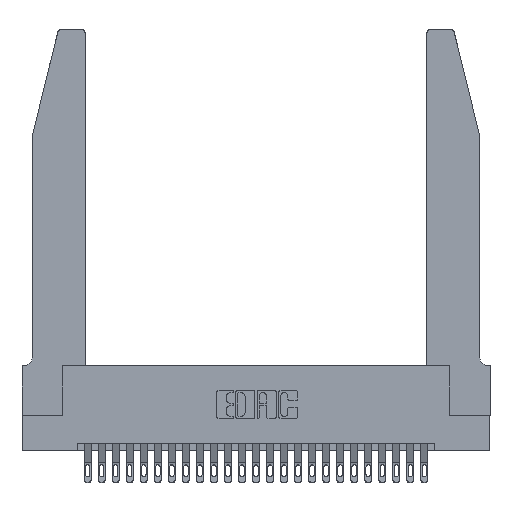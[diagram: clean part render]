
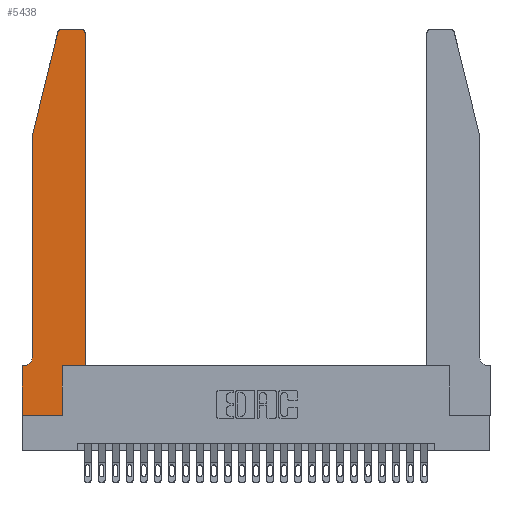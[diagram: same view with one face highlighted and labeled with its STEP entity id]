
A CAD part, top view. The second image highlights one B-rep face of the part: STEP entity #5438.
In plain terms, the highlighted planar face has unit normal (0, 0, 1).
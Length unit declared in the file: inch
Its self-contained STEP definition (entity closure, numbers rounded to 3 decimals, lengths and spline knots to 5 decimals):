
#113 = EDGE_CURVE ( 'NONE', #25436, #23786, #5286, .T. ) ;
#147 = EDGE_CURVE ( 'NONE', #23786, #20704, #4611, .T. ) ;
#660 = CARTESIAN_POINT ( 'NONE',  ( 0.284, 2.75, 0.37 ) ) ;
#758 = VECTOR ( 'NONE', #20936, 39.37008 ) ;
#1079 = PLANE ( 'NONE',  #24748 ) ;
#1210 = VERTEX_POINT ( 'NONE', #26761 ) ;
#1295 = AXIS2_PLACEMENT_3D ( 'NONE', #12065, #11718, #9719 ) ;
#1422 = FACE_OUTER_BOUND ( 'NONE', #10379, .T. ) ;
#1890 = VERTEX_POINT ( 'NONE', #9913 ) ;
#2035 = ORIENTED_EDGE ( 'NONE', *, *, #22057, .T. ) ;
#2702 = LINE ( 'NONE', #21032, #758 ) ;
#2763 = DIRECTION ( 'NONE',  ( 0., 1., 0. ) ) ;
#2892 = CARTESIAN_POINT ( 'NONE',  ( 0., 0., 0.37 ) ) ;
#3364 = ORIENTED_EDGE ( 'NONE', *, *, #16850, .T. ) ;
#3591 = DIRECTION ( 'NONE',  ( -1., 0., 0. ) ) ;
#3679 = CARTESIAN_POINT ( 'NONE',  ( 0., 0., 0.37 ) ) ;
#3851 = DIRECTION ( 'NONE',  ( 1., 0., 0. ) ) ;
#3941 = DIRECTION ( 'NONE',  ( 0., 0., 1. ) ) ;
#4061 = LINE ( 'NONE', #22363, #6693 ) ;
#4368 = LINE ( 'NONE', #18089, #11891 ) ;
#4611 = LINE ( 'NONE', #3679, #24851 ) ;
#5286 = LINE ( 'NONE', #16263, #26804 ) ;
#5438 = ADVANCED_FACE ( 'NONE', ( #1422 ), #1079, .T. ) ;
#6693 = VECTOR ( 'NONE', #19968, 39.37008 ) ;
#6712 = VECTOR ( 'NONE', #13705, 39.37008 ) ;
#7265 = ORIENTED_EDGE ( 'NONE', *, *, #12050, .T. ) ;
#7304 = CARTESIAN_POINT ( 'NONE',  ( 0.2865, 0., 0.37 ) ) ;
#7962 = CARTESIAN_POINT ( 'NONE',  ( 0.2865, 0.35, 0.37 ) ) ;
#8316 = CARTESIAN_POINT ( 'NONE',  ( 0.0755, 2., 0.37 ) ) ;
#8392 = VERTEX_POINT ( 'NONE', #660 ) ;
#9274 = CIRCLE ( 'NONE', #1295, 0.07 ) ;
#9284 = CARTESIAN_POINT ( 'NONE',  ( 0., 0.35, 0.37 ) ) ;
#9291 = DIRECTION ( 'NONE',  ( 1., 0., 0. ) ) ;
#9356 = EDGE_CURVE ( 'NONE', #17501, #8392, #16219, .T. ) ;
#9461 = DIRECTION ( 'NONE',  ( 1., 0., 0. ) ) ;
#9602 = VERTEX_POINT ( 'NONE', #13536 ) ;
#9719 = DIRECTION ( 'NONE',  ( -1., 0., 0. ) ) ;
#9913 = CARTESIAN_POINT ( 'NONE',  ( 0.0755, 2., 0.37 ) ) ;
#9938 = LINE ( 'NONE', #15140, #16427 ) ;
#10162 = CARTESIAN_POINT ( 'NONE',  ( 0.4205, 2.72, 0.37 ) ) ;
#10234 = CIRCLE ( 'NONE', #24543, 0.03 ) ;
#10379 = EDGE_LOOP ( 'NONE', ( #18372, #12619, #7265, #15109, #2035, #25795, #15486, #26771, #3364, #12554, #19840, #25245 ) ) ;
#10765 = VERTEX_POINT ( 'NONE', #7962 ) ;
#11630 = CARTESIAN_POINT ( 'NONE',  ( 0.0755, 2., 0.37 ) ) ;
#11718 = DIRECTION ( 'NONE',  ( 0., 0., -1. ) ) ;
#11820 = CARTESIAN_POINT ( 'NONE',  ( 0.0055, 0.35, 0.37 ) ) ;
#11891 = VECTOR ( 'NONE', #22448, 39.37008 ) ;
#12050 = EDGE_CURVE ( 'NONE', #9602, #1890, #23351, .T. ) ;
#12065 = CARTESIAN_POINT ( 'NONE',  ( 0.0055, 0.42, 0.37 ) ) ;
#12495 = EDGE_CURVE ( 'NONE', #1210, #14931, #9938, .T. ) ;
#12554 = ORIENTED_EDGE ( 'NONE', *, *, #21561, .T. ) ;
#12619 = ORIENTED_EDGE ( 'NONE', *, *, #13758, .T. ) ;
#12656 = VECTOR ( 'NONE', #12910, 39.37008 ) ;
#12910 = DIRECTION ( 'NONE',  ( -1., 0., 0. ) ) ;
#13092 = CARTESIAN_POINT ( 'NONE',  ( 0.2605, 2.75, 0.37 ) ) ;
#13536 = CARTESIAN_POINT ( 'NONE',  ( 0.25487, 2.72718, 0.37 ) ) ;
#13632 = DIRECTION ( 'NONE',  ( 0., 0., 1. ) ) ;
#13705 = DIRECTION ( 'NONE',  ( -0.239, -0.971, 0. ) ) ;
#13758 = EDGE_CURVE ( 'NONE', #8392, #9602, #10234, .T. ) ;
#14931 = VERTEX_POINT ( 'NONE', #19431 ) ;
#15109 = ORIENTED_EDGE ( 'NONE', *, *, #22905, .T. ) ;
#15140 = CARTESIAN_POINT ( 'NONE',  ( 0.4505, 0.35, 0.37 ) ) ;
#15486 = ORIENTED_EDGE ( 'NONE', *, *, #147, .T. ) ;
#15714 = DIRECTION ( 'NONE',  ( 0., 0., 1. ) ) ;
#16219 = LINE ( 'NONE', #13092, #12656 ) ;
#16263 = CARTESIAN_POINT ( 'NONE',  ( 0.0755, 0.35, 0.37 ) ) ;
#16415 = VERTEX_POINT ( 'NONE', #7304 ) ;
#16427 = VECTOR ( 'NONE', #2763, 39.37008 ) ;
#16850 = EDGE_CURVE ( 'NONE', #16415, #10765, #2702, .T. ) ;
#17501 = VERTEX_POINT ( 'NONE', #18637 ) ;
#17822 = VECTOR ( 'NONE', #22817, 39.37008 ) ;
#18089 = CARTESIAN_POINT ( 'NONE',  ( 0.4505, 0.35, 0.37 ) ) ;
#18372 = ORIENTED_EDGE ( 'NONE', *, *, #9356, .T. ) ;
#18637 = CARTESIAN_POINT ( 'NONE',  ( 0.4205, 2.75, 0.37 ) ) ;
#18761 = VERTEX_POINT ( 'NONE', #25028 ) ;
#19119 = AXIS2_PLACEMENT_3D ( 'NONE', #10162, #3941, #3851 ) ;
#19431 = CARTESIAN_POINT ( 'NONE',  ( 0.4505, 2.72, 0.37 ) ) ;
#19840 = ORIENTED_EDGE ( 'NONE', *, *, #12495, .T. ) ;
#19968 = DIRECTION ( 'NONE',  ( 1., 0., 0. ) ) ;
#20704 = VERTEX_POINT ( 'NONE', #2892 ) ;
#20936 = DIRECTION ( 'NONE',  ( 0., 1., 0. ) ) ;
#21032 = CARTESIAN_POINT ( 'NONE',  ( 0.2865, 0.35, 0.37 ) ) ;
#21454 = EDGE_CURVE ( 'NONE', #20704, #16415, #4061, .T. ) ;
#21561 = EDGE_CURVE ( 'NONE', #10765, #1210, #4368, .T. ) ;
#21776 = CARTESIAN_POINT ( 'NONE',  ( 0.284, 2.72, 0.37 ) ) ;
#22057 = EDGE_CURVE ( 'NONE', #18761, #25436, #9274, .T. ) ;
#22363 = CARTESIAN_POINT ( 'NONE',  ( 0., 0., 0.37 ) ) ;
#22448 = DIRECTION ( 'NONE',  ( 1., 0., 0. ) ) ;
#22681 = DIRECTION ( 'NONE',  ( 0., -1., 0. ) ) ;
#22817 = DIRECTION ( 'NONE',  ( 0., -1., 0. ) ) ;
#22905 = EDGE_CURVE ( 'NONE', #1890, #18761, #26264, .T. ) ;
#23351 = LINE ( 'NONE', #11630, #6712 ) ;
#23678 = CARTESIAN_POINT ( 'NONE',  ( 0., 0.35, 0.37 ) ) ;
#23786 = VERTEX_POINT ( 'NONE', #23678 ) ;
#24008 = EDGE_CURVE ( 'NONE', #14931, #17501, #25578, .T. ) ;
#24543 = AXIS2_PLACEMENT_3D ( 'NONE', #21776, #13632, #9291 ) ;
#24748 = AXIS2_PLACEMENT_3D ( 'NONE', #9284, #15714, #9461 ) ;
#24851 = VECTOR ( 'NONE', #22681, 39.37008 ) ;
#25028 = CARTESIAN_POINT ( 'NONE',  ( 0.0755, 0.42, 0.37 ) ) ;
#25245 = ORIENTED_EDGE ( 'NONE', *, *, #24008, .T. ) ;
#25436 = VERTEX_POINT ( 'NONE', #11820 ) ;
#25578 = CIRCLE ( 'NONE', #19119, 0.03 ) ;
#25795 = ORIENTED_EDGE ( 'NONE', *, *, #113, .T. ) ;
#26264 = LINE ( 'NONE', #8316, #17822 ) ;
#26761 = CARTESIAN_POINT ( 'NONE',  ( 0.4505, 0.35, 0.37 ) ) ;
#26771 = ORIENTED_EDGE ( 'NONE', *, *, #21454, .T. ) ;
#26804 = VECTOR ( 'NONE', #3591, 39.37008 ) ;
